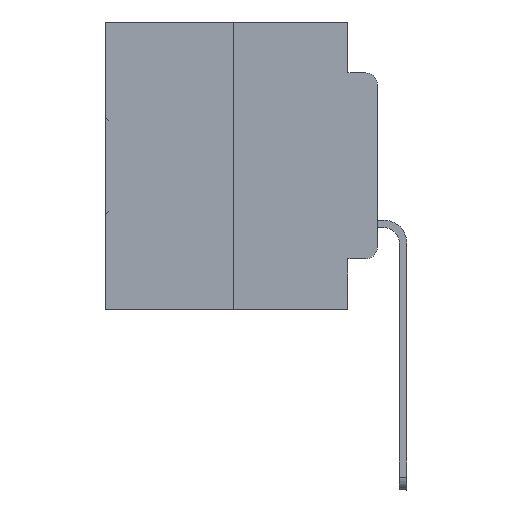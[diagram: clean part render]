
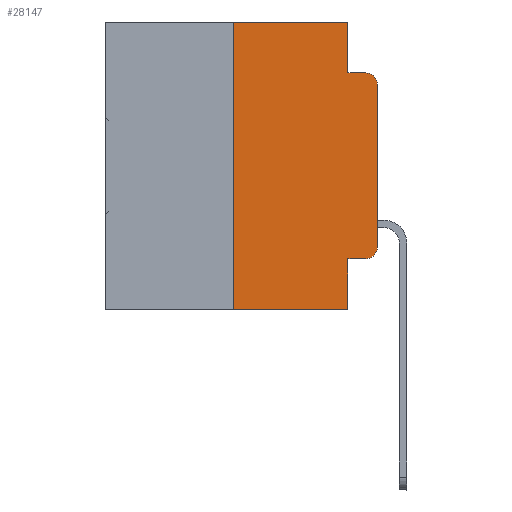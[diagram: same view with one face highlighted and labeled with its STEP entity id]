
A CAD part, left-side view. The second image highlights one B-rep face of the part: STEP entity #28147.
In plain terms, the highlighted planar face has unit normal (-1, 0, 0).
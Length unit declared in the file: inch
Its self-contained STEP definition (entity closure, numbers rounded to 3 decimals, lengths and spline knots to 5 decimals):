
#980 = VERTEX_POINT ( 'NONE', #16537 ) ;
#1273 = LINE ( 'NONE', #24710, #4087 ) ;
#2291 = CARTESIAN_POINT ( 'NONE',  ( 0., 0.051, 0. ) ) ;
#2633 = CARTESIAN_POINT ( 'NONE',  ( 0., 0.25, 0. ) ) ;
#3469 = DIRECTION ( 'NONE',  ( 0., -1., 0. ) ) ;
#3478 = DIRECTION ( 'NONE',  ( 0., 0., -1. ) ) ;
#3528 = ORIENTED_EDGE ( 'NONE', *, *, #10975, .T. ) ;
#3690 = ORIENTED_EDGE ( 'NONE', *, *, #13508, .T. ) ;
#4087 = VECTOR ( 'NONE', #32405, 39.37008 ) ;
#4116 = CARTESIAN_POINT ( 'NONE',  ( 0., 0.051, -0.0885 ) ) ;
#4184 = CARTESIAN_POINT ( 'NONE',  ( 0., 0., -0.1085 ) ) ;
#4458 = DIRECTION ( 'NONE',  ( 0., 0., -1. ) ) ;
#4611 = LINE ( 'NONE', #26192, #18922 ) ;
#4948 = AXIS2_PLACEMENT_3D ( 'NONE', #30167, #12501, #15037 ) ;
#5114 = EDGE_CURVE ( 'NONE', #980, #5533, #17462, .T. ) ;
#5533 = VERTEX_POINT ( 'NONE', #25816 ) ;
#5922 = VERTEX_POINT ( 'NONE', #2291 ) ;
#6947 = EDGE_CURVE ( 'NONE', #8818, #980, #15787, .T. ) ;
#7153 = CARTESIAN_POINT ( 'NONE',  ( 0., 0.25, -0.5 ) ) ;
#8523 = VERTEX_POINT ( 'NONE', #24982 ) ;
#8704 = AXIS2_PLACEMENT_3D ( 'NONE', #31256, #28705, #18595 ) ;
#8818 = VERTEX_POINT ( 'NONE', #10633 ) ;
#9078 = VECTOR ( 'NONE', #21755, 39.37008 ) ;
#9164 = VECTOR ( 'NONE', #20388, 39.37008 ) ;
#9273 = VERTEX_POINT ( 'NONE', #7153 ) ;
#9447 = LINE ( 'NONE', #4116, #19377 ) ;
#9837 = CARTESIAN_POINT ( 'NONE',  ( 0., 0.473, -0.5 ) ) ;
#10178 = LINE ( 'NONE', #24058, #31613 ) ;
#10633 = CARTESIAN_POINT ( 'NONE',  ( 0., 0.051, -0.4115 ) ) ;
#10890 = CARTESIAN_POINT ( 'NONE',  ( 0., 0.473, 0. ) ) ;
#10975 = EDGE_CURVE ( 'NONE', #5533, #16821, #1273, .T. ) ;
#11257 = ORIENTED_EDGE ( 'NONE', *, *, #6947, .T. ) ;
#11459 = CARTESIAN_POINT ( 'NONE',  ( 0., 0.02, -0.3915 ) ) ;
#12091 = EDGE_CURVE ( 'NONE', #9273, #8523, #15076, .T. ) ;
#12312 = ORIENTED_EDGE ( 'NONE', *, *, #14574, .F. ) ;
#12501 = DIRECTION ( 'NONE',  ( 1., 0., 0. ) ) ;
#13508 = EDGE_CURVE ( 'NONE', #16821, #18509, #24514, .T. ) ;
#14574 = EDGE_CURVE ( 'NONE', #8818, #23454, #10178, .T. ) ;
#15037 = DIRECTION ( 'NONE',  ( 0., 0., -1. ) ) ;
#15076 = LINE ( 'NONE', #2633, #9164 ) ;
#15224 = ORIENTED_EDGE ( 'NONE', *, *, #32511, .T. ) ;
#15363 = EDGE_LOOP ( 'NONE', ( #3528, #3690, #26734, #28324, #30804, #18712, #15224, #12312, #11257, #17039 ) ) ;
#15402 = VERTEX_POINT ( 'NONE', #20464 ) ;
#15670 = EDGE_CURVE ( 'NONE', #8523, #5922, #15933, .T. ) ;
#15787 = LINE ( 'NONE', #31734, #9078 ) ;
#15933 = LINE ( 'NONE', #10890, #25445 ) ;
#16537 = CARTESIAN_POINT ( 'NONE',  ( 0., 0.02, -0.4115 ) ) ;
#16821 = VERTEX_POINT ( 'NONE', #4184 ) ;
#17039 = ORIENTED_EDGE ( 'NONE', *, *, #5114, .T. ) ;
#17043 = CARTESIAN_POINT ( 'NONE',  ( 0., 0.02, -0.0885 ) ) ;
#17462 = CIRCLE ( 'NONE', #22860, 0.02 ) ;
#17866 = EDGE_CURVE ( 'NONE', #15402, #18509, #9447, .T. ) ;
#18509 = VERTEX_POINT ( 'NONE', #17043 ) ;
#18595 = DIRECTION ( 'NONE',  ( 0., 0., -1. ) ) ;
#18712 = ORIENTED_EDGE ( 'NONE', *, *, #12091, .F. ) ;
#18922 = VECTOR ( 'NONE', #3478, 39.37008 ) ;
#19377 = VECTOR ( 'NONE', #21869, 39.37008 ) ;
#19721 = DIRECTION ( 'NONE',  ( 0., -1., 0. ) ) ;
#19961 = PLANE ( 'NONE',  #4948 ) ;
#20388 = DIRECTION ( 'NONE',  ( 0., 0., 1. ) ) ;
#20464 = CARTESIAN_POINT ( 'NONE',  ( 0., 0.051, -0.0885 ) ) ;
#21755 = DIRECTION ( 'NONE',  ( 0., -1., 0. ) ) ;
#21869 = DIRECTION ( 'NONE',  ( 0., -1., 0. ) ) ;
#22860 = AXIS2_PLACEMENT_3D ( 'NONE', #11459, #29241, #4458 ) ;
#23454 = VERTEX_POINT ( 'NONE', #31551 ) ;
#23518 = FACE_OUTER_BOUND ( 'NONE', #15363, .T. ) ;
#24058 = CARTESIAN_POINT ( 'NONE',  ( 0., 0.051, 0. ) ) ;
#24468 = LINE ( 'NONE', #9837, #31666 ) ;
#24514 = CIRCLE ( 'NONE', #8704, 0.02 ) ;
#24710 = CARTESIAN_POINT ( 'NONE',  ( 0., 0., 0. ) ) ;
#24982 = CARTESIAN_POINT ( 'NONE',  ( 0., 0.25, 0. ) ) ;
#25445 = VECTOR ( 'NONE', #3469, 39.37008 ) ;
#25816 = CARTESIAN_POINT ( 'NONE',  ( 0., 0., -0.3915 ) ) ;
#26192 = CARTESIAN_POINT ( 'NONE',  ( 0., 0.051, 0. ) ) ;
#26624 = DIRECTION ( 'NONE',  ( 0., 0., -1. ) ) ;
#26734 = ORIENTED_EDGE ( 'NONE', *, *, #17866, .F. ) ;
#28147 = ADVANCED_FACE ( 'NONE', ( #23518 ), #19961, .F. ) ;
#28324 = ORIENTED_EDGE ( 'NONE', *, *, #32859, .F. ) ;
#28705 = DIRECTION ( 'NONE',  ( -1., 0., 0. ) ) ;
#29241 = DIRECTION ( 'NONE',  ( -1., 0., 0. ) ) ;
#30167 = CARTESIAN_POINT ( 'NONE',  ( 0., 0.473, 0. ) ) ;
#30804 = ORIENTED_EDGE ( 'NONE', *, *, #15670, .F. ) ;
#31256 = CARTESIAN_POINT ( 'NONE',  ( 0., 0.02, -0.1085 ) ) ;
#31551 = CARTESIAN_POINT ( 'NONE',  ( 0., 0.051, -0.5 ) ) ;
#31613 = VECTOR ( 'NONE', #26624, 39.37008 ) ;
#31666 = VECTOR ( 'NONE', #19721, 39.37008 ) ;
#31734 = CARTESIAN_POINT ( 'NONE',  ( 0., 0.051, -0.4115 ) ) ;
#32405 = DIRECTION ( 'NONE',  ( 0., 0., 1. ) ) ;
#32511 = EDGE_CURVE ( 'NONE', #9273, #23454, #24468, .T. ) ;
#32859 = EDGE_CURVE ( 'NONE', #5922, #15402, #4611, .T. ) ;
